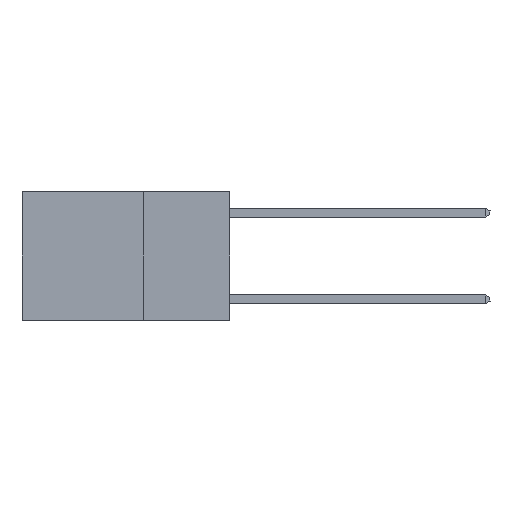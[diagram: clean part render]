
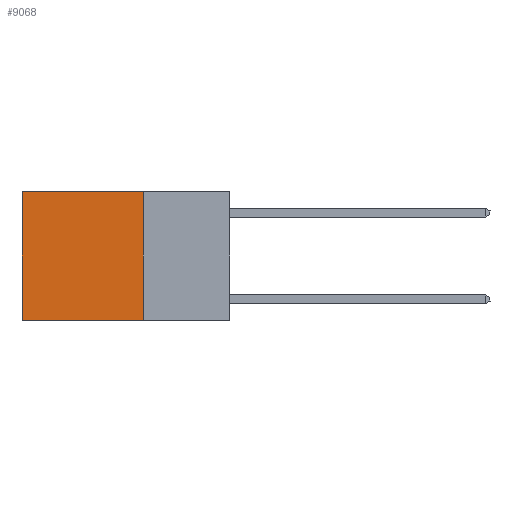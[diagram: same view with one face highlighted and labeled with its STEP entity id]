
A CAD part, left-side view. The second image highlights one B-rep face of the part: STEP entity #9068.
In plain terms, the highlighted planar face has unit normal (-1, 0, 0).
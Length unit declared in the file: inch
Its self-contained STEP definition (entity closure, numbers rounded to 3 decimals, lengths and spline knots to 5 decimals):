
#184 = CARTESIAN_POINT ( 'NONE',  ( 0.2625, 0.6, -0.37 ) ) ;
#440 = CARTESIAN_POINT ( 'NONE',  ( 0.2625, 0.25, 0. ) ) ;
#937 = ORIENTED_EDGE ( 'NONE', *, *, #11656, .F. ) ;
#1258 = VERTEX_POINT ( 'NONE', #7363 ) ;
#1710 = ORIENTED_EDGE ( 'NONE', *, *, #2845, .T. ) ;
#2280 = DIRECTION ( 'NONE',  ( 0., 1., 0. ) ) ;
#2384 = CARTESIAN_POINT ( 'NONE',  ( 0.2625, 0.25, 0. ) ) ;
#2459 = LINE ( 'NONE', #11966, #4443 ) ;
#2517 = EDGE_CURVE ( 'NONE', #7975, #6558, #5021, .T. ) ;
#2721 = VERTEX_POINT ( 'NONE', #184 ) ;
#2762 = ORIENTED_EDGE ( 'NONE', *, *, #2517, .F. ) ;
#2845 = EDGE_CURVE ( 'NONE', #7975, #1258, #9799, .T. ) ;
#2902 = PLANE ( 'NONE',  #9379 ) ;
#3480 = ORIENTED_EDGE ( 'NONE', *, *, #9071, .T. ) ;
#4443 = VECTOR ( 'NONE', #13176, 39.37008 ) ;
#5021 = LINE ( 'NONE', #8197, #10802 ) ;
#5032 = FACE_OUTER_BOUND ( 'NONE', #8339, .T. ) ;
#5582 = DIRECTION ( 'NONE',  ( 0., 1., 0. ) ) ;
#6558 = VERTEX_POINT ( 'NONE', #13419 ) ;
#6650 = CARTESIAN_POINT ( 'NONE',  ( 0.2625, 0.25, 0. ) ) ;
#6784 = DIRECTION ( 'NONE',  ( 1., 0., 0. ) ) ;
#7363 = CARTESIAN_POINT ( 'NONE',  ( 0.2625, 0.6, 0. ) ) ;
#7671 = CARTESIAN_POINT ( 'NONE',  ( 0.2625, 0.25, -0.37 ) ) ;
#7713 = DIRECTION ( 'NONE',  ( 0., 0., -1. ) ) ;
#7975 = VERTEX_POINT ( 'NONE', #440 ) ;
#8197 = CARTESIAN_POINT ( 'NONE',  ( 0.2625, 0.25, 0. ) ) ;
#8339 = EDGE_LOOP ( 'NONE', ( #3480, #937, #2762, #1710 ) ) ;
#8475 = VECTOR ( 'NONE', #2280, 39.37008 ) ;
#9068 = ADVANCED_FACE ( 'NONE', ( #5032 ), #2902, .F. ) ;
#9071 = EDGE_CURVE ( 'NONE', #1258, #2721, #2459, .T. ) ;
#9379 = AXIS2_PLACEMENT_3D ( 'NONE', #2384, #6784, #7713 ) ;
#9687 = VECTOR ( 'NONE', #5582, 39.37008 ) ;
#9799 = LINE ( 'NONE', #6650, #9687 ) ;
#10103 = DIRECTION ( 'NONE',  ( 0., 0., -1. ) ) ;
#10802 = VECTOR ( 'NONE', #10103, 39.37008 ) ;
#10809 = LINE ( 'NONE', #7671, #8475 ) ;
#11656 = EDGE_CURVE ( 'NONE', #6558, #2721, #10809, .T. ) ;
#11966 = CARTESIAN_POINT ( 'NONE',  ( 0.2625, 0.6, 0. ) ) ;
#13176 = DIRECTION ( 'NONE',  ( 0., 0., -1. ) ) ;
#13419 = CARTESIAN_POINT ( 'NONE',  ( 0.2625, 0.25, -0.37 ) ) ;
